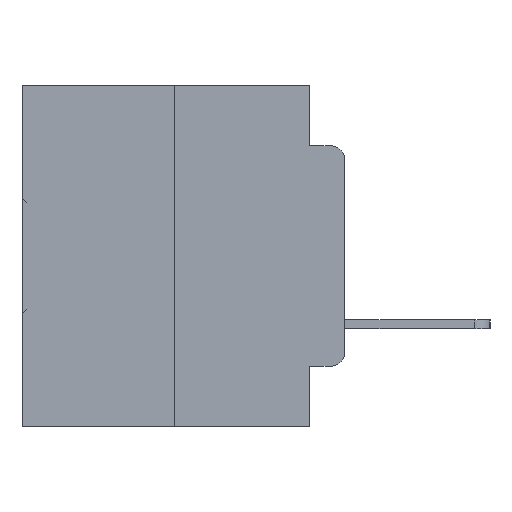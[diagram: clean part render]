
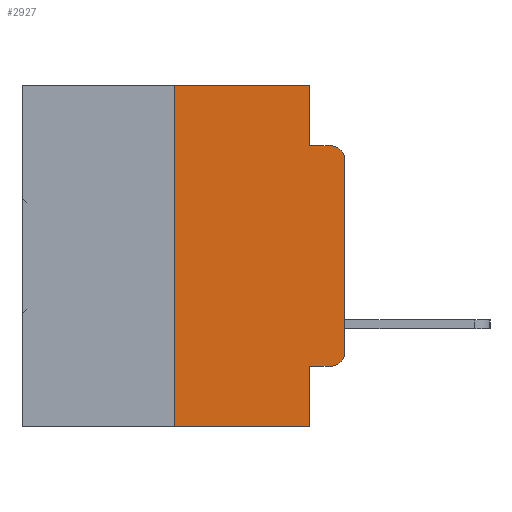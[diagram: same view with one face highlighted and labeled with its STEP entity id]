
A CAD part, left-side view. The second image highlights one B-rep face of the part: STEP entity #2927.
In plain terms, the highlighted planar face has unit normal (-1, 0, 0).
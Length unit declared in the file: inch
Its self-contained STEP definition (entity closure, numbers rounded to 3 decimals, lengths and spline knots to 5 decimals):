
#121 = EDGE_CURVE ( 'NONE', #3458, #4006, #15980, .T. ) ;
#186 = DIRECTION ( 'NONE',  ( 0., -1., 0. ) ) ;
#999 = CARTESIAN_POINT ( 'NONE',  ( 0., 0.051, -0.4115 ) ) ;
#1481 = CARTESIAN_POINT ( 'NONE',  ( 0., 0.02, -0.4115 ) ) ;
#1779 = LINE ( 'NONE', #18130, #7640 ) ;
#1815 = VERTEX_POINT ( 'NONE', #22020 ) ;
#1854 = CARTESIAN_POINT ( 'NONE',  ( 0., 0.473, 0. ) ) ;
#1943 = ORIENTED_EDGE ( 'NONE', *, *, #30004, .F. ) ;
#2089 = CARTESIAN_POINT ( 'NONE',  ( 0., 0.051, -0.0885 ) ) ;
#2333 = ORIENTED_EDGE ( 'NONE', *, *, #4768, .F. ) ;
#2350 = VERTEX_POINT ( 'NONE', #2089 ) ;
#2916 = EDGE_CURVE ( 'NONE', #1815, #14707, #3943, .T. ) ;
#2927 = ADVANCED_FACE ( 'NONE', ( #28428 ), #16067, .F. ) ;
#3458 = VERTEX_POINT ( 'NONE', #7210 ) ;
#3529 = CARTESIAN_POINT ( 'NONE',  ( 0., 0.473, -0.5 ) ) ;
#3534 = EDGE_LOOP ( 'NONE', ( #10880, #25395, #2333, #10516, #17747, #25763, #27267, #1943, #3537, #5119 ) ) ;
#3537 = ORIENTED_EDGE ( 'NONE', *, *, #22558, .T. ) ;
#3943 = LINE ( 'NONE', #3529, #17021 ) ;
#4006 = VERTEX_POINT ( 'NONE', #23519 ) ;
#4152 = EDGE_CURVE ( 'NONE', #4006, #21205, #18122, .T. ) ;
#4376 = DIRECTION ( 'NONE',  ( 0., -1., 0. ) ) ;
#4768 = EDGE_CURVE ( 'NONE', #2350, #21205, #24208, .T. ) ;
#5119 = ORIENTED_EDGE ( 'NONE', *, *, #28015, .T. ) ;
#5623 = DIRECTION ( 'NONE',  ( 0., 0., -1. ) ) ;
#7210 = CARTESIAN_POINT ( 'NONE',  ( 0., 0., -0.3915 ) ) ;
#7416 = LINE ( 'NONE', #1854, #11660 ) ;
#7640 = VECTOR ( 'NONE', #27932, 39.37008 ) ;
#9425 = LINE ( 'NONE', #28355, #14421 ) ;
#9504 = CARTESIAN_POINT ( 'NONE',  ( 0., 0.25, 0. ) ) ;
#9730 = VECTOR ( 'NONE', #31240, 39.37008 ) ;
#9766 = VECTOR ( 'NONE', #5623, 39.37008 ) ;
#10249 = CARTESIAN_POINT ( 'NONE',  ( 0., 0.051, -0.0885 ) ) ;
#10516 = ORIENTED_EDGE ( 'NONE', *, *, #25097, .F. ) ;
#10532 = DIRECTION ( 'NONE',  ( -1., 0., 0. ) ) ;
#10880 = ORIENTED_EDGE ( 'NONE', *, *, #121, .T. ) ;
#11660 = VECTOR ( 'NONE', #4376, 39.37008 ) ;
#12941 = AXIS2_PLACEMENT_3D ( 'NONE', #25143, #10532, #27557 ) ;
#13086 = AXIS2_PLACEMENT_3D ( 'NONE', #28118, #13331, #25281 ) ;
#13331 = DIRECTION ( 'NONE',  ( 1., 0., 0. ) ) ;
#14348 = CARTESIAN_POINT ( 'NONE',  ( 0., 0.02, -0.1085 ) ) ;
#14421 = VECTOR ( 'NONE', #16149, 39.37008 ) ;
#14707 = VERTEX_POINT ( 'NONE', #26175 ) ;
#15299 = EDGE_CURVE ( 'NONE', #1815, #27043, #1779, .T. ) ;
#15498 = CARTESIAN_POINT ( 'NONE',  ( 0., 0.051, 0. ) ) ;
#15980 = LINE ( 'NONE', #21237, #22472 ) ;
#16067 = PLANE ( 'NONE',  #13086 ) ;
#16149 = DIRECTION ( 'NONE',  ( 0., -1., 0. ) ) ;
#16287 = CARTESIAN_POINT ( 'NONE',  ( 0., 0.02, -0.0885 ) ) ;
#16781 = DIRECTION ( 'NONE',  ( 0., 0., -1. ) ) ;
#17021 = VECTOR ( 'NONE', #19063, 39.37008 ) ;
#17747 = ORIENTED_EDGE ( 'NONE', *, *, #18310, .F. ) ;
#18122 = CIRCLE ( 'NONE', #28544, 0.02 ) ;
#18130 = CARTESIAN_POINT ( 'NONE',  ( 0., 0.25, 0. ) ) ;
#18310 = EDGE_CURVE ( 'NONE', #27043, #22987, #7416, .T. ) ;
#19063 = DIRECTION ( 'NONE',  ( 0., -1., 0. ) ) ;
#20212 = CIRCLE ( 'NONE', #12941, 0.02 ) ;
#21205 = VERTEX_POINT ( 'NONE', #16287 ) ;
#21237 = CARTESIAN_POINT ( 'NONE',  ( 0., 0., 0. ) ) ;
#21318 = DIRECTION ( 'NONE',  ( 0., 0., 1. ) ) ;
#21771 = VERTEX_POINT ( 'NONE', #999 ) ;
#22020 = CARTESIAN_POINT ( 'NONE',  ( 0., 0.25, -0.5 ) ) ;
#22472 = VECTOR ( 'NONE', #21318, 39.37008 ) ;
#22558 = EDGE_CURVE ( 'NONE', #21771, #28169, #9425, .T. ) ;
#22692 = VECTOR ( 'NONE', #186, 39.37008 ) ;
#22728 = CARTESIAN_POINT ( 'NONE',  ( 0., 0.051, 0. ) ) ;
#22987 = VERTEX_POINT ( 'NONE', #22728 ) ;
#23491 = LINE ( 'NONE', #26528, #9730 ) ;
#23519 = CARTESIAN_POINT ( 'NONE',  ( 0., 0., -0.1085 ) ) ;
#23526 = LINE ( 'NONE', #15498, #9766 ) ;
#24208 = LINE ( 'NONE', #10249, #22692 ) ;
#25097 = EDGE_CURVE ( 'NONE', #22987, #2350, #23526, .T. ) ;
#25143 = CARTESIAN_POINT ( 'NONE',  ( 0., 0.02, -0.3915 ) ) ;
#25281 = DIRECTION ( 'NONE',  ( 0., 0., -1. ) ) ;
#25395 = ORIENTED_EDGE ( 'NONE', *, *, #4152, .T. ) ;
#25763 = ORIENTED_EDGE ( 'NONE', *, *, #15299, .F. ) ;
#26175 = CARTESIAN_POINT ( 'NONE',  ( 0., 0.051, -0.5 ) ) ;
#26528 = CARTESIAN_POINT ( 'NONE',  ( 0., 0.051, 0. ) ) ;
#27043 = VERTEX_POINT ( 'NONE', #9504 ) ;
#27267 = ORIENTED_EDGE ( 'NONE', *, *, #2916, .T. ) ;
#27557 = DIRECTION ( 'NONE',  ( 0., 0., -1. ) ) ;
#27932 = DIRECTION ( 'NONE',  ( 0., 0., 1. ) ) ;
#28015 = EDGE_CURVE ( 'NONE', #28169, #3458, #20212, .T. ) ;
#28118 = CARTESIAN_POINT ( 'NONE',  ( 0., 0.473, 0. ) ) ;
#28169 = VERTEX_POINT ( 'NONE', #1481 ) ;
#28355 = CARTESIAN_POINT ( 'NONE',  ( 0., 0.051, -0.4115 ) ) ;
#28428 = FACE_OUTER_BOUND ( 'NONE', #3534, .T. ) ;
#28544 = AXIS2_PLACEMENT_3D ( 'NONE', #14348, #31271, #16781 ) ;
#30004 = EDGE_CURVE ( 'NONE', #21771, #14707, #23491, .T. ) ;
#31240 = DIRECTION ( 'NONE',  ( 0., 0., -1. ) ) ;
#31271 = DIRECTION ( 'NONE',  ( -1., 0., 0. ) ) ;
